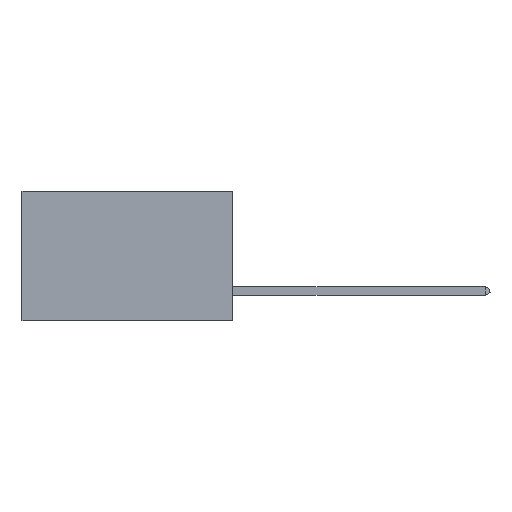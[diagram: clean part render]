
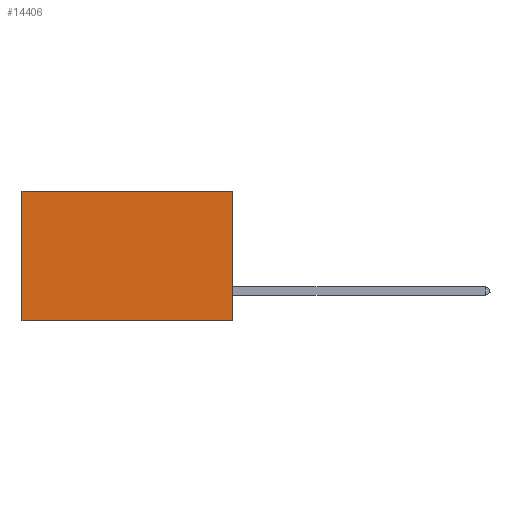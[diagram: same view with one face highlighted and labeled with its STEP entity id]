
A CAD part, left-side view. The second image highlights one B-rep face of the part: STEP entity #14406.
In plain terms, the highlighted planar face has unit normal (-1, 0, 0).
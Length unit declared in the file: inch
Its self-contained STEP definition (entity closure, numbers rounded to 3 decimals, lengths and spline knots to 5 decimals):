
#636 = CARTESIAN_POINT ( 'NONE',  ( 0.2875, 0., 0. ) ) ;
#1189 = EDGE_CURVE ( 'NONE', #44275, #43170, #7796, .T. ) ;
#1398 = DIRECTION ( 'NONE',  ( 0., 0., -1. ) ) ;
#2220 = CARTESIAN_POINT ( 'NONE',  ( 0.2875, 0., -0.37 ) ) ;
#4251 = ORIENTED_EDGE ( 'NONE', *, *, #33957, .F. ) ;
#6785 = EDGE_CURVE ( 'NONE', #9178, #7119, #37683, .T. ) ;
#7119 = VERTEX_POINT ( 'NONE', #13567 ) ;
#7796 = LINE ( 'NONE', #23348, #23827 ) ;
#9178 = VERTEX_POINT ( 'NONE', #636 ) ;
#9717 = VECTOR ( 'NONE', #28330, 39.37008 ) ;
#9822 = ORIENTED_EDGE ( 'NONE', *, *, #39342, .T. ) ;
#13567 = CARTESIAN_POINT ( 'NONE',  ( 0.2875, 0., -0.37 ) ) ;
#14406 = ADVANCED_FACE ( 'NONE', ( #27433 ), #19533, .F. ) ;
#16208 = ORIENTED_EDGE ( 'NONE', *, *, #6785, .F. ) ;
#18748 = AXIS2_PLACEMENT_3D ( 'NONE', #45075, #37871, #1398 ) ;
#19533 = PLANE ( 'NONE',  #18748 ) ;
#20174 = ORIENTED_EDGE ( 'NONE', *, *, #1189, .T. ) ;
#20735 = DIRECTION ( 'NONE',  ( 0., 1., 0. ) ) ;
#22272 = VECTOR ( 'NONE', #20735, 39.37008 ) ;
#23348 = CARTESIAN_POINT ( 'NONE',  ( 0.2875, 0.6, 0. ) ) ;
#23827 = VECTOR ( 'NONE', #26579, 39.37008 ) ;
#26579 = DIRECTION ( 'NONE',  ( 0., 0., -1. ) ) ;
#26752 = EDGE_LOOP ( 'NONE', ( #20174, #4251, #16208, #9822 ) ) ;
#27433 = FACE_OUTER_BOUND ( 'NONE', #26752, .T. ) ;
#27444 = VECTOR ( 'NONE', #43062, 39.37008 ) ;
#28330 = DIRECTION ( 'NONE',  ( 0., 1., 0. ) ) ;
#28541 = CARTESIAN_POINT ( 'NONE',  ( 0.2875, 0., 0. ) ) ;
#31981 = LINE ( 'NONE', #28541, #22272 ) ;
#33957 = EDGE_CURVE ( 'NONE', #7119, #43170, #36596, .T. ) ;
#36596 = LINE ( 'NONE', #2220, #9717 ) ;
#37683 = LINE ( 'NONE', #47221, #27444 ) ;
#37871 = DIRECTION ( 'NONE',  ( 1., 0., 0. ) ) ;
#39342 = EDGE_CURVE ( 'NONE', #9178, #44275, #31981, .T. ) ;
#43062 = DIRECTION ( 'NONE',  ( 0., 0., -1. ) ) ;
#43170 = VERTEX_POINT ( 'NONE', #43530 ) ;
#43530 = CARTESIAN_POINT ( 'NONE',  ( 0.2875, 0.6, -0.37 ) ) ;
#44275 = VERTEX_POINT ( 'NONE', #46604 ) ;
#45075 = CARTESIAN_POINT ( 'NONE',  ( 0.2875, 0., 0. ) ) ;
#46604 = CARTESIAN_POINT ( 'NONE',  ( 0.2875, 0.6, 0. ) ) ;
#47221 = CARTESIAN_POINT ( 'NONE',  ( 0.2875, 0., 0. ) ) ;
